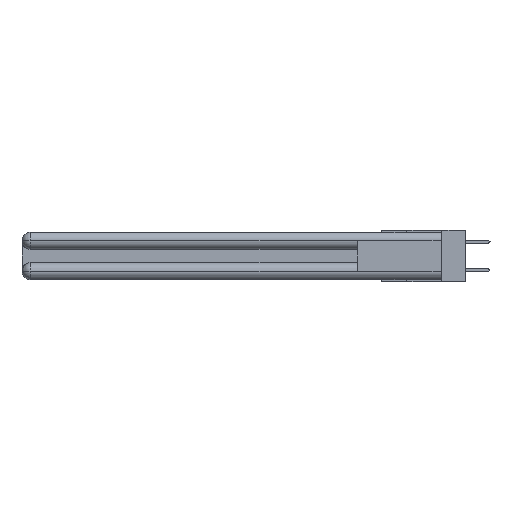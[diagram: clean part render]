
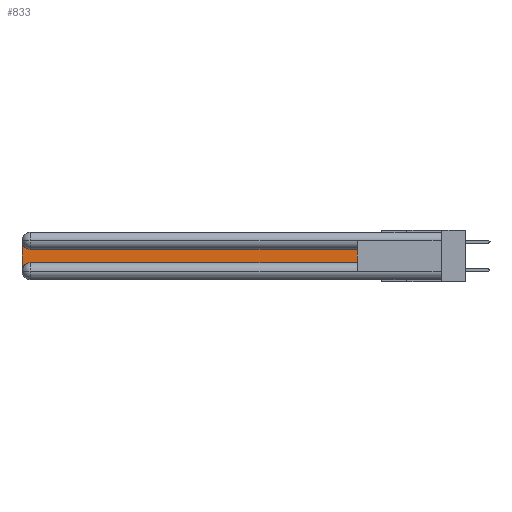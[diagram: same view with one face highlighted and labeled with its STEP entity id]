
A CAD part, left-side view. The second image highlights one B-rep face of the part: STEP entity #833.
In plain terms, the highlighted planar face has unit normal (-1, 0, 0).
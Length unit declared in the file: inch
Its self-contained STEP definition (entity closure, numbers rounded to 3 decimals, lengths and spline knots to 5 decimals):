
#238 = DIRECTION ( 'NONE',  ( 0., 0., -1. ) ) ;
#281 = DIRECTION ( 'NONE',  ( 0., 0., 1. ) ) ;
#414 = VERTEX_POINT ( 'NONE', #1671 ) ;
#833 = ADVANCED_FACE ( 'NONE', ( #29076 ), #21924, .F. ) ;
#1129 = ORIENTED_EDGE ( 'NONE', *, *, #5060, .T. ) ;
#1263 = ORIENTED_EDGE ( 'NONE', *, *, #29836, .T. ) ;
#1671 = CARTESIAN_POINT ( 'NONE',  ( 0.075, 2.94, -0.2175 ) ) ;
#3064 = DIRECTION ( 'NONE',  ( 1., 0., 0. ) ) ;
#3173 = DIRECTION ( 'NONE',  ( 0., 0., -1. ) ) ;
#5060 = EDGE_CURVE ( 'NONE', #15077, #25373, #29597, .T. ) ;
#5808 = CARTESIAN_POINT ( 'NONE',  ( 0.075, 0.6, -0.2175 ) ) ;
#10047 = LINE ( 'NONE', #13227, #31512 ) ;
#10734 = CARTESIAN_POINT ( 'NONE',  ( 0.075, 3., -0.2175 ) ) ;
#11859 = CARTESIAN_POINT ( 'NONE',  ( 0.075, 3., -0.2775 ) ) ;
#12202 = VERTEX_POINT ( 'NONE', #11859 ) ;
#12249 = CIRCLE ( 'NONE', #12562, 0.06 ) ;
#12562 = AXIS2_PLACEMENT_3D ( 'NONE', #19008, #16844, #14015 ) ;
#13227 = CARTESIAN_POINT ( 'NONE',  ( 0.075, 0.6, -0.2175 ) ) ;
#13341 = EDGE_CURVE ( 'NONE', #25373, #12202, #26079, .T. ) ;
#13670 = ORIENTED_EDGE ( 'NONE', *, *, #13341, .T. ) ;
#14015 = DIRECTION ( 'NONE',  ( 0., 0., -1. ) ) ;
#15077 = VERTEX_POINT ( 'NONE', #22336 ) ;
#16844 = DIRECTION ( 'NONE',  ( 1., 0., 0. ) ) ;
#17075 = CARTESIAN_POINT ( 'NONE',  ( 0.075, 0.6, -0.1225 ) ) ;
#17665 = EDGE_CURVE ( 'NONE', #31079, #22904, #10047, .T. ) ;
#18161 = LINE ( 'NONE', #5808, #26216 ) ;
#19008 = CARTESIAN_POINT ( 'NONE',  ( 0.075, 2.94, -0.2775 ) ) ;
#19282 = LINE ( 'NONE', #32171, #23698 ) ;
#19629 = VECTOR ( 'NONE', #238, 39.37008 ) ;
#20918 = ORIENTED_EDGE ( 'NONE', *, *, #17665, .T. ) ;
#21262 = ORIENTED_EDGE ( 'NONE', *, *, #27015, .T. ) ;
#21924 = PLANE ( 'NONE',  #24755 ) ;
#22336 = CARTESIAN_POINT ( 'NONE',  ( 0.075, 2.94, -0.1225 ) ) ;
#22837 = EDGE_LOOP ( 'NONE', ( #21262, #1129, #13670, #1263, #26714, #20918 ) ) ;
#22904 = VERTEX_POINT ( 'NONE', #17075 ) ;
#23698 = VECTOR ( 'NONE', #27041, 39.37008 ) ;
#24755 = AXIS2_PLACEMENT_3D ( 'NONE', #27028, #32478, #27130 ) ;
#25373 = VERTEX_POINT ( 'NONE', #25394 ) ;
#25394 = CARTESIAN_POINT ( 'NONE',  ( 0.075, 3., -0.0625 ) ) ;
#25586 = EDGE_CURVE ( 'NONE', #414, #31079, #18161, .T. ) ;
#26079 = LINE ( 'NONE', #10734, #19629 ) ;
#26216 = VECTOR ( 'NONE', #26836, 39.37008 ) ;
#26714 = ORIENTED_EDGE ( 'NONE', *, *, #25586, .T. ) ;
#26836 = DIRECTION ( 'NONE',  ( 0., -1., 0. ) ) ;
#27015 = EDGE_CURVE ( 'NONE', #22904, #15077, #19282, .T. ) ;
#27028 = CARTESIAN_POINT ( 'NONE',  ( 0.075, 3., -0.1225 ) ) ;
#27041 = DIRECTION ( 'NONE',  ( 0., 1., 0. ) ) ;
#27130 = DIRECTION ( 'NONE',  ( 0., 0., -1. ) ) ;
#29016 = CARTESIAN_POINT ( 'NONE',  ( 0.075, 2.94, -0.0625 ) ) ;
#29076 = FACE_OUTER_BOUND ( 'NONE', #22837, .T. ) ;
#29099 = CARTESIAN_POINT ( 'NONE',  ( 0.075, 0.6, -0.2175 ) ) ;
#29597 = CIRCLE ( 'NONE', #31761, 0.06 ) ;
#29836 = EDGE_CURVE ( 'NONE', #12202, #414, #12249, .T. ) ;
#31079 = VERTEX_POINT ( 'NONE', #29099 ) ;
#31512 = VECTOR ( 'NONE', #281, 39.37008 ) ;
#31761 = AXIS2_PLACEMENT_3D ( 'NONE', #29016, #3064, #3173 ) ;
#32171 = CARTESIAN_POINT ( 'NONE',  ( 0.075, 0.6, -0.1225 ) ) ;
#32478 = DIRECTION ( 'NONE',  ( 1., 0., 0. ) ) ;
